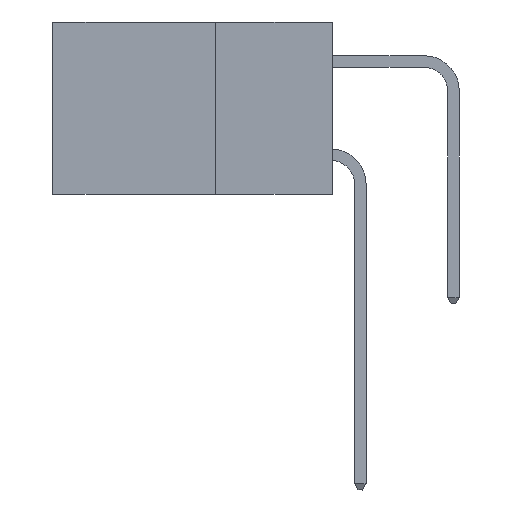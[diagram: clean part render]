
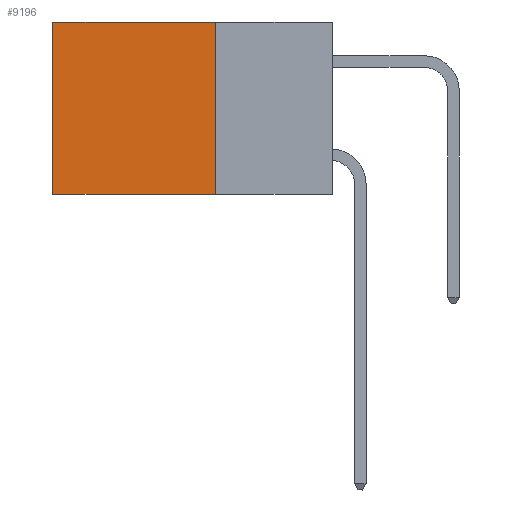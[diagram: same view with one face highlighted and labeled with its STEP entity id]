
A CAD part, left-side view. The second image highlights one B-rep face of the part: STEP entity #9196.
In plain terms, the highlighted planar face has unit normal (-1, 0, 0).
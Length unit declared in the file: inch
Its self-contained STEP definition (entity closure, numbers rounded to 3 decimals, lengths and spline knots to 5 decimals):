
#1315 = CARTESIAN_POINT ( 'NONE',  ( 0.2615, 0.25, -0.37 ) ) ;
#1779 = VERTEX_POINT ( 'NONE', #9995 ) ;
#1953 = ORIENTED_EDGE ( 'NONE', *, *, #11550, .F. ) ;
#2352 = ORIENTED_EDGE ( 'NONE', *, *, #17196, .T. ) ;
#3337 = DIRECTION ( 'NONE',  ( 1., 0., 0. ) ) ;
#3511 = CARTESIAN_POINT ( 'NONE',  ( 0.2615, 0.25, -0.37 ) ) ;
#3536 = VECTOR ( 'NONE', #8340, 39.37008 ) ;
#4350 = FACE_OUTER_BOUND ( 'NONE', #6337, .T. ) ;
#5754 = VECTOR ( 'NONE', #12069, 39.37008 ) ;
#6337 = EDGE_LOOP ( 'NONE', ( #2352, #1953, #23749, #14711 ) ) ;
#7007 = LINE ( 'NONE', #21424, #5754 ) ;
#8340 = DIRECTION ( 'NONE',  ( 0., 1., 0. ) ) ;
#8805 = LINE ( 'NONE', #19788, #3536 ) ;
#9196 = ADVANCED_FACE ( 'NONE', ( #4350 ), #24277, .F. ) ;
#9628 = VERTEX_POINT ( 'NONE', #16072 ) ;
#9995 = CARTESIAN_POINT ( 'NONE',  ( 0.2615, 0.25, -0.37 ) ) ;
#10094 = DIRECTION ( 'NONE',  ( 0., 0., -1. ) ) ;
#11449 = DIRECTION ( 'NONE',  ( 0., 0., -1. ) ) ;
#11550 = EDGE_CURVE ( 'NONE', #1779, #21724, #7007, .T. ) ;
#11617 = CARTESIAN_POINT ( 'NONE',  ( 0.2615, 0.6, -0.37 ) ) ;
#11763 = CARTESIAN_POINT ( 'NONE',  ( 0.2615, 0.25, 0. ) ) ;
#12069 = DIRECTION ( 'NONE',  ( 0., 1., 0. ) ) ;
#12745 = EDGE_CURVE ( 'NONE', #16574, #9628, #8805, .T. ) ;
#13916 = AXIS2_PLACEMENT_3D ( 'NONE', #1315, #3337, #16912 ) ;
#14711 = ORIENTED_EDGE ( 'NONE', *, *, #12745, .T. ) ;
#15212 = LINE ( 'NONE', #3511, #19043 ) ;
#15238 = LINE ( 'NONE', #23239, #24533 ) ;
#16072 = CARTESIAN_POINT ( 'NONE',  ( 0.2615, 0.6, 0. ) ) ;
#16574 = VERTEX_POINT ( 'NONE', #11763 ) ;
#16912 = DIRECTION ( 'NONE',  ( 0., 0., -1. ) ) ;
#17196 = EDGE_CURVE ( 'NONE', #9628, #21724, #15238, .T. ) ;
#17674 = EDGE_CURVE ( 'NONE', #16574, #1779, #15212, .T. ) ;
#19043 = VECTOR ( 'NONE', #11449, 39.37008 ) ;
#19788 = CARTESIAN_POINT ( 'NONE',  ( 0.2615, 0.25, 0. ) ) ;
#21424 = CARTESIAN_POINT ( 'NONE',  ( 0.2615, 0.25, -0.37 ) ) ;
#21724 = VERTEX_POINT ( 'NONE', #11617 ) ;
#23239 = CARTESIAN_POINT ( 'NONE',  ( 0.2615, 0.6, -0.37 ) ) ;
#23749 = ORIENTED_EDGE ( 'NONE', *, *, #17674, .F. ) ;
#24277 = PLANE ( 'NONE',  #13916 ) ;
#24533 = VECTOR ( 'NONE', #10094, 39.37008 ) ;
